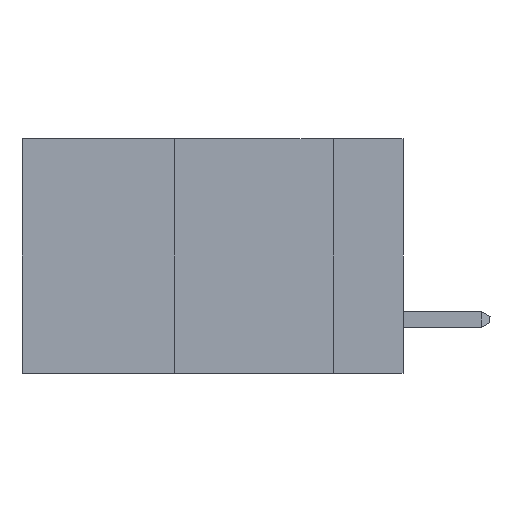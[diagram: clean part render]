
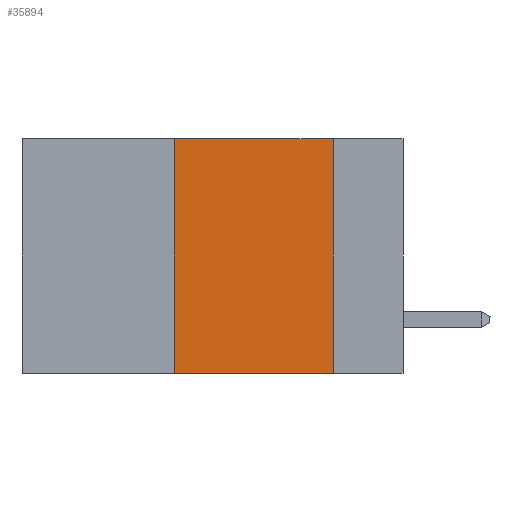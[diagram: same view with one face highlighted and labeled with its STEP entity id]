
A CAD part, left-side view. The second image highlights one B-rep face of the part: STEP entity #35894.
In plain terms, the highlighted planar face has unit normal (-1, 0, 0).
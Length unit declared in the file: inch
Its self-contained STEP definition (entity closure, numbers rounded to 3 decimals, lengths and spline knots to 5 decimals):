
#906 = DIRECTION ( 'NONE',  ( 0., 0., -1. ) ) ;
#1050 = VECTOR ( 'NONE', #31819, 39.37008 ) ;
#1218 = DIRECTION ( 'NONE',  ( 1., 0., 0. ) ) ;
#1892 = EDGE_CURVE ( 'NONE', #7726, #37220, #45267, .T. ) ;
#3790 = FACE_OUTER_BOUND ( 'NONE', #29741, .T. ) ;
#5388 = AXIS2_PLACEMENT_3D ( 'NONE', #12125, #1218, #906 ) ;
#7726 = VERTEX_POINT ( 'NONE', #12410 ) ;
#9452 = EDGE_CURVE ( 'NONE', #14377, #37220, #21402, .T. ) ;
#12125 = CARTESIAN_POINT ( 'NONE',  ( 0., 0.6, 0. ) ) ;
#12410 = CARTESIAN_POINT ( 'NONE',  ( 0., 0.11, 0. ) ) ;
#13837 = VECTOR ( 'NONE', #28913, 39.37008 ) ;
#14377 = VERTEX_POINT ( 'NONE', #24593 ) ;
#14503 = CARTESIAN_POINT ( 'NONE',  ( 0., 0.11, -0.37 ) ) ;
#15627 = ORIENTED_EDGE ( 'NONE', *, *, #46635, .F. ) ;
#17299 = EDGE_CURVE ( 'NONE', #28572, #7726, #23547, .T. ) ;
#18712 = CARTESIAN_POINT ( 'NONE',  ( 0., 0.6, 0. ) ) ;
#20975 = DIRECTION ( 'NONE',  ( 0., 0., -1. ) ) ;
#21402 = LINE ( 'NONE', #28100, #45840 ) ;
#23547 = LINE ( 'NONE', #18712, #13837 ) ;
#24593 = CARTESIAN_POINT ( 'NONE',  ( 0., 0.36, -0.37 ) ) ;
#28100 = CARTESIAN_POINT ( 'NONE',  ( 0., 0.6, -0.37 ) ) ;
#28572 = VERTEX_POINT ( 'NONE', #39433 ) ;
#28713 = DIRECTION ( 'NONE',  ( 0., -1., 0. ) ) ;
#28913 = DIRECTION ( 'NONE',  ( 0., -1., 0. ) ) ;
#29741 = EDGE_LOOP ( 'NONE', ( #46707, #42285, #15627, #31393 ) ) ;
#30125 = LINE ( 'NONE', #46466, #1050 ) ;
#31393 = ORIENTED_EDGE ( 'NONE', *, *, #9452, .T. ) ;
#31819 = DIRECTION ( 'NONE',  ( 0., 0., 1. ) ) ;
#35894 = ADVANCED_FACE ( 'NONE', ( #3790 ), #40554, .F. ) ;
#37220 = VERTEX_POINT ( 'NONE', #14503 ) ;
#38452 = CARTESIAN_POINT ( 'NONE',  ( 0., 0.11, 0. ) ) ;
#39433 = CARTESIAN_POINT ( 'NONE',  ( 0., 0.36, 0. ) ) ;
#40554 = PLANE ( 'NONE',  #5388 ) ;
#41815 = VECTOR ( 'NONE', #20975, 39.37008 ) ;
#42285 = ORIENTED_EDGE ( 'NONE', *, *, #17299, .F. ) ;
#45267 = LINE ( 'NONE', #38452, #41815 ) ;
#45840 = VECTOR ( 'NONE', #28713, 39.37008 ) ;
#46466 = CARTESIAN_POINT ( 'NONE',  ( 0., 0.36, 0. ) ) ;
#46635 = EDGE_CURVE ( 'NONE', #14377, #28572, #30125, .T. ) ;
#46707 = ORIENTED_EDGE ( 'NONE', *, *, #1892, .F. ) ;
